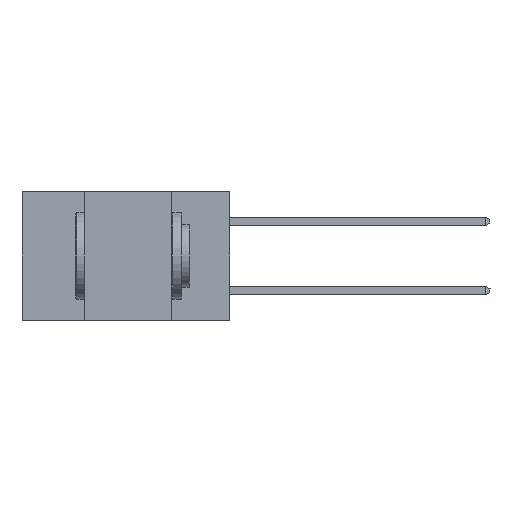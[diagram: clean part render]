
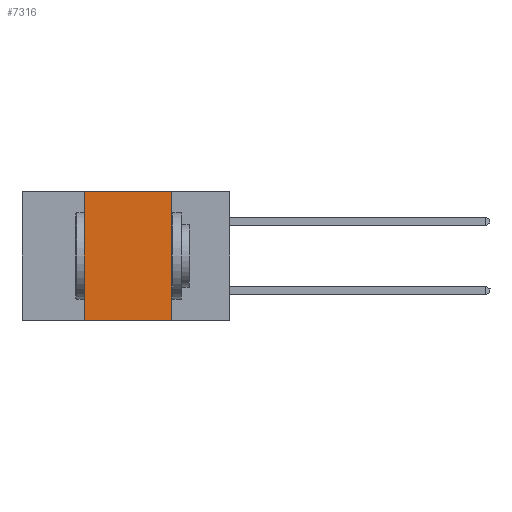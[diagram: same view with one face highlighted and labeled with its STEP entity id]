
A CAD part, left-side view. The second image highlights one B-rep face of the part: STEP entity #7316.
In plain terms, the highlighted planar face has unit normal (-1, 0, 0).
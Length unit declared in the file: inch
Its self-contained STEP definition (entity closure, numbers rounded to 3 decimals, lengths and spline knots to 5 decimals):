
#524 = EDGE_LOOP ( 'NONE', ( #2348, #17828, #22836, #13426 ) ) ;
#760 = LINE ( 'NONE', #15806, #15101 ) ;
#1178 = VERTEX_POINT ( 'NONE', #14773 ) ;
#1975 = CARTESIAN_POINT ( 'NONE',  ( 0., 0.17, -0.37 ) ) ;
#1990 = VECTOR ( 'NONE', #9745, 39.37008 ) ;
#2348 = ORIENTED_EDGE ( 'NONE', *, *, #10738, .F. ) ;
#2558 = EDGE_CURVE ( 'NONE', #12737, #13530, #760, .T. ) ;
#3357 = CARTESIAN_POINT ( 'NONE',  ( 0., 0.6, 0. ) ) ;
#4016 = VERTEX_POINT ( 'NONE', #20619 ) ;
#4108 = DIRECTION ( 'NONE',  ( 0., 0., 1. ) ) ;
#5584 = CARTESIAN_POINT ( 'NONE',  ( 0., 0.42, -0.37 ) ) ;
#6280 = DIRECTION ( 'NONE',  ( 0., -1., 0. ) ) ;
#6363 = CARTESIAN_POINT ( 'NONE',  ( 0., 0.6, 0. ) ) ;
#6412 = LINE ( 'NONE', #17184, #21374 ) ;
#6966 = EDGE_CURVE ( 'NONE', #12737, #4016, #6412, .T. ) ;
#7316 = ADVANCED_FACE ( 'NONE', ( #23123 ), #22098, .F. ) ;
#9480 = EDGE_CURVE ( 'NONE', #4016, #1178, #19297, .T. ) ;
#9745 = DIRECTION ( 'NONE',  ( 0., 0., -1. ) ) ;
#10738 = EDGE_CURVE ( 'NONE', #1178, #13530, #11900, .T. ) ;
#10877 = DIRECTION ( 'NONE',  ( 1., 0., 0. ) ) ;
#11900 = LINE ( 'NONE', #19088, #1990 ) ;
#12737 = VERTEX_POINT ( 'NONE', #5584 ) ;
#13426 = ORIENTED_EDGE ( 'NONE', *, *, #2558, .T. ) ;
#13530 = VERTEX_POINT ( 'NONE', #1975 ) ;
#14314 = VECTOR ( 'NONE', #6280, 39.37008 ) ;
#14773 = CARTESIAN_POINT ( 'NONE',  ( 0., 0.17, 0. ) ) ;
#15101 = VECTOR ( 'NONE', #23696, 39.37008 ) ;
#15806 = CARTESIAN_POINT ( 'NONE',  ( 0., 0.6, -0.37 ) ) ;
#17184 = CARTESIAN_POINT ( 'NONE',  ( 0., 0.42, -0.37 ) ) ;
#17545 = AXIS2_PLACEMENT_3D ( 'NONE', #3357, #10877, #24009 ) ;
#17828 = ORIENTED_EDGE ( 'NONE', *, *, #9480, .F. ) ;
#19088 = CARTESIAN_POINT ( 'NONE',  ( 0., 0.17, -0.37 ) ) ;
#19297 = LINE ( 'NONE', #6363, #14314 ) ;
#20619 = CARTESIAN_POINT ( 'NONE',  ( 0., 0.42, 0. ) ) ;
#21374 = VECTOR ( 'NONE', #4108, 39.37008 ) ;
#22098 = PLANE ( 'NONE',  #17545 ) ;
#22836 = ORIENTED_EDGE ( 'NONE', *, *, #6966, .F. ) ;
#23123 = FACE_OUTER_BOUND ( 'NONE', #524, .T. ) ;
#23696 = DIRECTION ( 'NONE',  ( 0., -1., 0. ) ) ;
#24009 = DIRECTION ( 'NONE',  ( 0., 0., -1. ) ) ;
